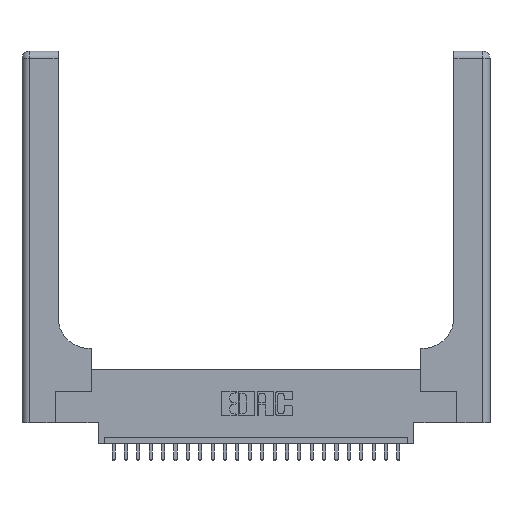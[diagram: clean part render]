
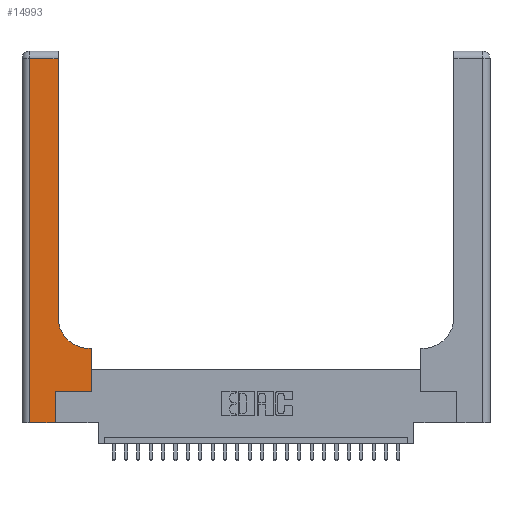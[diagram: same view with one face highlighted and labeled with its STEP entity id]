
A CAD part, top view. The second image highlights one B-rep face of the part: STEP entity #14993.
In plain terms, the highlighted planar face has unit normal (0, 0, 1).
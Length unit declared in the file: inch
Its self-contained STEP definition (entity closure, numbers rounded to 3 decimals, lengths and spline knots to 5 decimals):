
#606 = VECTOR ( 'NONE', #2449, 39.37008 ) ;
#660 = CARTESIAN_POINT ( 'NONE',  ( 0.2915, 0.85, 0.37 ) ) ;
#1115 = ORIENTED_EDGE ( 'NONE', *, *, #9069, .T. ) ;
#1348 = DIRECTION ( 'NONE',  ( -1., 0., 0. ) ) ;
#1878 = ORIENTED_EDGE ( 'NONE', *, *, #5604, .T. ) ;
#2094 = EDGE_CURVE ( 'NONE', #18444, #6502, #6872, .T. ) ;
#2449 = DIRECTION ( 'NONE',  ( 0., 1., 0. ) ) ;
#3065 = ORIENTED_EDGE ( 'NONE', *, *, #15355, .T. ) ;
#3272 = DIRECTION ( 'NONE',  ( 1., 0., 0. ) ) ;
#3393 = LINE ( 'NONE', #24369, #13699 ) ;
#3845 = DIRECTION ( 'NONE',  ( 0., -1., 0. ) ) ;
#4229 = VERTEX_POINT ( 'NONE', #13437 ) ;
#4377 = ORIENTED_EDGE ( 'NONE', *, *, #13374, .T. ) ;
#5377 = CARTESIAN_POINT ( 'NONE',  ( 0.06, 2.94, 0.37 ) ) ;
#5395 = DIRECTION ( 'NONE',  ( 0., 0., -1. ) ) ;
#5419 = CARTESIAN_POINT ( 'NONE',  ( 0.5585, 0.25, 0.37 ) ) ;
#5604 = EDGE_CURVE ( 'NONE', #4229, #15301, #9256, .T. ) ;
#5786 = CARTESIAN_POINT ( 'NONE',  ( 0.06, 0., 0.37 ) ) ;
#5964 = LINE ( 'NONE', #6788, #23042 ) ;
#6435 = AXIS2_PLACEMENT_3D ( 'NONE', #9572, #19525, #3272 ) ;
#6460 = DIRECTION ( 'NONE',  ( 1., 0., 0. ) ) ;
#6502 = VERTEX_POINT ( 'NONE', #5419 ) ;
#6521 = CARTESIAN_POINT ( 'NONE',  ( 0.5415, 0.6, 0.37 ) ) ;
#6707 = DIRECTION ( 'NONE',  ( -1., 0., 0. ) ) ;
#6788 = CARTESIAN_POINT ( 'NONE',  ( 0.2915, 0.6, 0.37 ) ) ;
#6872 = LINE ( 'NONE', #22193, #16842 ) ;
#7035 = VERTEX_POINT ( 'NONE', #25117 ) ;
#7724 = VERTEX_POINT ( 'NONE', #6521 ) ;
#7934 = VERTEX_POINT ( 'NONE', #660 ) ;
#8677 = ORIENTED_EDGE ( 'NONE', *, *, #23448, .T. ) ;
#9069 = EDGE_CURVE ( 'NONE', #6502, #7035, #25553, .T. ) ;
#9256 = LINE ( 'NONE', #24524, #12684 ) ;
#9572 = CARTESIAN_POINT ( 'NONE',  ( 0.5415, 0.85, 0.37 ) ) ;
#10550 = CARTESIAN_POINT ( 'NONE',  ( 0.269, 0., 0.37 ) ) ;
#10969 = DIRECTION ( 'NONE',  ( 0., 1., 0. ) ) ;
#11249 = ORIENTED_EDGE ( 'NONE', *, *, #14281, .T. ) ;
#11924 = LINE ( 'NONE', #18744, #18091 ) ;
#12684 = VECTOR ( 'NONE', #24768, 39.37008 ) ;
#12759 = CARTESIAN_POINT ( 'NONE',  ( 0.5585, 0.25, 0.37 ) ) ;
#13374 = EDGE_CURVE ( 'NONE', #20320, #18444, #11924, .T. ) ;
#13437 = CARTESIAN_POINT ( 'NONE',  ( 0.2915, 2.94, 0.37 ) ) ;
#13699 = VECTOR ( 'NONE', #6460, 39.37008 ) ;
#14266 = FACE_OUTER_BOUND ( 'NONE', #21447, .T. ) ;
#14281 = EDGE_CURVE ( 'NONE', #15301, #20118, #16187, .T. ) ;
#14518 = ORIENTED_EDGE ( 'NONE', *, *, #18786, .T. ) ;
#14721 = CARTESIAN_POINT ( 'NONE',  ( 0.2915, 3., 0.37 ) ) ;
#14993 = ADVANCED_FACE ( 'NONE', ( #14266 ), #21109, .F. ) ;
#15301 = VERTEX_POINT ( 'NONE', #5377 ) ;
#15355 = EDGE_CURVE ( 'NONE', #7724, #7934, #16730, .T. ) ;
#15857 = VECTOR ( 'NONE', #16377, 39.37008 ) ;
#16187 = LINE ( 'NONE', #16894, #19887 ) ;
#16377 = DIRECTION ( 'NONE',  ( 0., 1., 0. ) ) ;
#16730 = CIRCLE ( 'NONE', #6435, 0.25 ) ;
#16842 = VECTOR ( 'NONE', #23937, 39.37008 ) ;
#16894 = CARTESIAN_POINT ( 'NONE',  ( 0.06, 3., 0.37 ) ) ;
#18091 = VECTOR ( 'NONE', #10969, 39.37008 ) ;
#18444 = VERTEX_POINT ( 'NONE', #25266 ) ;
#18744 = CARTESIAN_POINT ( 'NONE',  ( 0.269, 0., 0.37 ) ) ;
#18786 = EDGE_CURVE ( 'NONE', #7934, #4229, #20784, .T. ) ;
#19185 = CARTESIAN_POINT ( 'NONE',  ( 0., 3., 0.37 ) ) ;
#19278 = ORIENTED_EDGE ( 'NONE', *, *, #2094, .T. ) ;
#19525 = DIRECTION ( 'NONE',  ( 0., 0., -1. ) ) ;
#19887 = VECTOR ( 'NONE', #3845, 39.37008 ) ;
#20118 = VERTEX_POINT ( 'NONE', #5786 ) ;
#20320 = VERTEX_POINT ( 'NONE', #10550 ) ;
#20784 = LINE ( 'NONE', #14721, #15857 ) ;
#20853 = ORIENTED_EDGE ( 'NONE', *, *, #25211, .T. ) ;
#21109 = PLANE ( 'NONE',  #22890 ) ;
#21447 = EDGE_LOOP ( 'NONE', ( #14518, #1878, #11249, #20853, #4377, #19278, #1115, #8677, #3065 ) ) ;
#22193 = CARTESIAN_POINT ( 'NONE',  ( 0.269, 0.25, 0.37 ) ) ;
#22890 = AXIS2_PLACEMENT_3D ( 'NONE', #19185, #5395, #1348 ) ;
#23042 = VECTOR ( 'NONE', #6707, 39.37008 ) ;
#23448 = EDGE_CURVE ( 'NONE', #7035, #7724, #5964, .T. ) ;
#23937 = DIRECTION ( 'NONE',  ( 1., 0., 0. ) ) ;
#24369 = CARTESIAN_POINT ( 'NONE',  ( 0., 0., 0.37 ) ) ;
#24524 = CARTESIAN_POINT ( 'NONE',  ( 0., 2.94, 0.37 ) ) ;
#24768 = DIRECTION ( 'NONE',  ( -1., 0., 0. ) ) ;
#25117 = CARTESIAN_POINT ( 'NONE',  ( 0.5585, 0.6, 0.37 ) ) ;
#25211 = EDGE_CURVE ( 'NONE', #20118, #20320, #3393, .T. ) ;
#25266 = CARTESIAN_POINT ( 'NONE',  ( 0.269, 0.25, 0.37 ) ) ;
#25553 = LINE ( 'NONE', #12759, #606 ) ;
